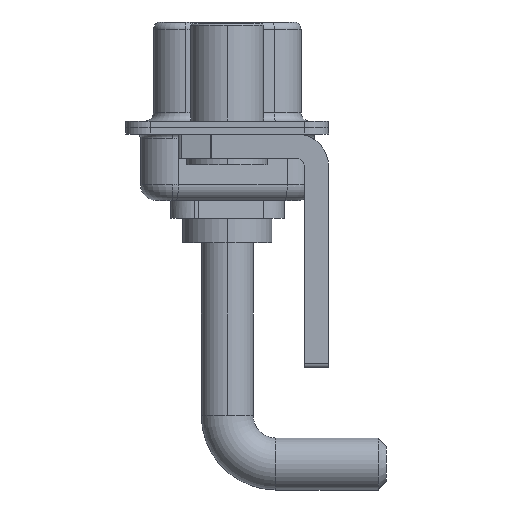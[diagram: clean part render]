
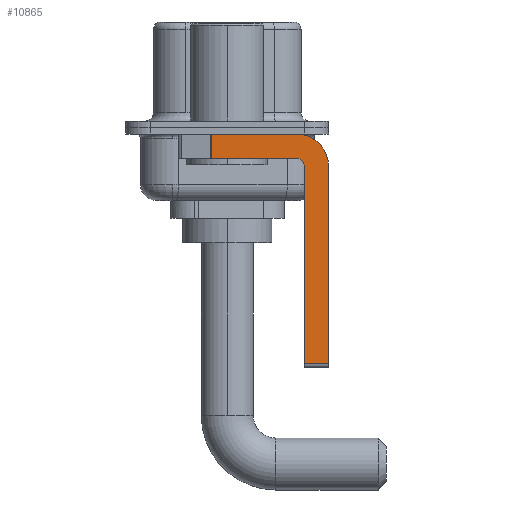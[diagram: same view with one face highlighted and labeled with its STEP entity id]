
A CAD part, left-side view. The second image highlights one B-rep face of the part: STEP entity #10865.
In plain terms, the highlighted planar face has unit normal (-1, 0, 0).
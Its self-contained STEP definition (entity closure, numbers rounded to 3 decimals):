
#286 = ORIENTED_EDGE ( 'NONE', *, *, #7784, .F. ) ;
#525 = LINE ( 'NONE', #16100, #8571 ) ;
#528 = VECTOR ( 'NONE', #1597, 1000. ) ;
#668 = EDGE_CURVE ( 'NONE', #10101, #3947, #9954, .T. ) ;
#982 = CARTESIAN_POINT ( 'NONE',  ( -2.9, -6.25, -14.55 ) ) ;
#1012 = ORIENTED_EDGE ( 'NONE', *, *, #9337, .F. ) ;
#1343 = DIRECTION ( 'NONE',  ( 1., 0., 0. ) ) ;
#1569 = ORIENTED_EDGE ( 'NONE', *, *, #9967, .F. ) ;
#1597 = DIRECTION ( 'NONE',  ( 0., 1., 0. ) ) ;
#1860 = AXIS2_PLACEMENT_3D ( 'NONE', #2185, #2363, #9991 ) ;
#2100 = CARTESIAN_POINT ( 'NONE',  ( -2.9, 0.978, -1.9 ) ) ;
#2185 = CARTESIAN_POINT ( 'NONE',  ( -2.9, -4.25, -2.4 ) ) ;
#2301 = CARTESIAN_POINT ( 'NONE',  ( -2.9, -4.25, -2.4 ) ) ;
#2363 = DIRECTION ( 'NONE',  ( -1., 0., 0. ) ) ;
#2443 = LINE ( 'NONE', #2100, #6920 ) ;
#2919 = VERTEX_POINT ( 'NONE', #982 ) ;
#3410 = CARTESIAN_POINT ( 'NONE',  ( -2.9, -4.25, -1.9 ) ) ;
#3825 = VERTEX_POINT ( 'NONE', #15152 ) ;
#3947 = VERTEX_POINT ( 'NONE', #10360 ) ;
#4152 = DIRECTION ( 'NONE',  ( 0., 0., 1. ) ) ;
#5175 = CARTESIAN_POINT ( 'NONE',  ( -2.9, -6.25, -2.4 ) ) ;
#5517 = ORIENTED_EDGE ( 'NONE', *, *, #668, .F. ) ;
#5588 = AXIS2_PLACEMENT_3D ( 'NONE', #7871, #1343, #6664 ) ;
#5749 = DIRECTION ( 'NONE',  ( 0., -1., 0. ) ) ;
#5906 = FACE_OUTER_BOUND ( 'NONE', #9325, .T. ) ;
#6664 = DIRECTION ( 'NONE',  ( 0., 0., -1. ) ) ;
#6813 = LINE ( 'NONE', #11774, #15966 ) ;
#6920 = VECTOR ( 'NONE', #12887, 1000. ) ;
#7396 = EDGE_CURVE ( 'NONE', #3825, #2919, #8668, .T. ) ;
#7613 = ORIENTED_EDGE ( 'NONE', *, *, #16662, .F. ) ;
#7784 = EDGE_CURVE ( 'NONE', #14571, #13018, #12133, .T. ) ;
#7871 = CARTESIAN_POINT ( 'NONE',  ( -2.9, -4.25, -2.4 ) ) ;
#8571 = VECTOR ( 'NONE', #5749, 1000. ) ;
#8578 = DIRECTION ( 'NONE',  ( 0., -1., 0. ) ) ;
#8668 = LINE ( 'NONE', #11402, #10978 ) ;
#8755 = CARTESIAN_POINT ( 'NONE',  ( -2.9, -4.75, -2.4 ) ) ;
#9325 = EDGE_LOOP ( 'NONE', ( #11924, #14016, #286, #1012, #7613, #14814, #1569, #5517 ) ) ;
#9337 = EDGE_CURVE ( 'NONE', #10302, #14571, #16624, .T. ) ;
#9339 = CARTESIAN_POINT ( 'NONE',  ( -2.9, 0.978, -0.4 ) ) ;
#9358 = DIRECTION ( 'NONE',  ( 0., 0., -1. ) ) ;
#9498 = CARTESIAN_POINT ( 'NONE',  ( -2.9, 0.978, -1.9 ) ) ;
#9954 = CIRCLE ( 'NONE', #5588, 2. ) ;
#9967 = EDGE_CURVE ( 'NONE', #3947, #2919, #10391, .T. ) ;
#9971 = VECTOR ( 'NONE', #9358, 1000. ) ;
#9991 = DIRECTION ( 'NONE',  ( 0., 0., 1. ) ) ;
#10101 = VERTEX_POINT ( 'NONE', #13703 ) ;
#10302 = VERTEX_POINT ( 'NONE', #8755 ) ;
#10360 = CARTESIAN_POINT ( 'NONE',  ( -2.9, -6.25, -2.4 ) ) ;
#10391 = LINE ( 'NONE', #5175, #9971 ) ;
#10402 = VERTEX_POINT ( 'NONE', #9339 ) ;
#10607 = CARTESIAN_POINT ( 'NONE',  ( -2.9, -4.25, -1.9 ) ) ;
#10865 = ADVANCED_FACE ( 'NONE', ( #5906 ), #14031, .F. ) ;
#10978 = VECTOR ( 'NONE', #8578, 1000. ) ;
#11227 = AXIS2_PLACEMENT_3D ( 'NONE', #2301, #13856, #12749 ) ;
#11402 = CARTESIAN_POINT ( 'NONE',  ( -2.9, -4.25, -14.55 ) ) ;
#11774 = CARTESIAN_POINT ( 'NONE',  ( -2.9, -4.75, -14.8 ) ) ;
#11924 = ORIENTED_EDGE ( 'NONE', *, *, #15952, .F. ) ;
#12133 = LINE ( 'NONE', #10607, #528 ) ;
#12749 = DIRECTION ( 'NONE',  ( 0., 0., -1. ) ) ;
#12887 = DIRECTION ( 'NONE',  ( 0., 0., -1. ) ) ;
#13018 = VERTEX_POINT ( 'NONE', #9498 ) ;
#13703 = CARTESIAN_POINT ( 'NONE',  ( -2.9, -4.25, -0.4 ) ) ;
#13729 = EDGE_CURVE ( 'NONE', #10402, #13018, #2443, .T. ) ;
#13856 = DIRECTION ( 'NONE',  ( 1., 0., 0. ) ) ;
#14016 = ORIENTED_EDGE ( 'NONE', *, *, #13729, .T. ) ;
#14031 = PLANE ( 'NONE',  #11227 ) ;
#14571 = VERTEX_POINT ( 'NONE', #3410 ) ;
#14814 = ORIENTED_EDGE ( 'NONE', *, *, #7396, .T. ) ;
#15152 = CARTESIAN_POINT ( 'NONE',  ( -2.9, -4.75, -14.55 ) ) ;
#15952 = EDGE_CURVE ( 'NONE', #10402, #10101, #525, .T. ) ;
#15966 = VECTOR ( 'NONE', #4152, 1000. ) ;
#16100 = CARTESIAN_POINT ( 'NONE',  ( -2.9, 3., -0.4 ) ) ;
#16624 = CIRCLE ( 'NONE', #1860, 0.5 ) ;
#16662 = EDGE_CURVE ( 'NONE', #3825, #10302, #6813, .T. ) ;
